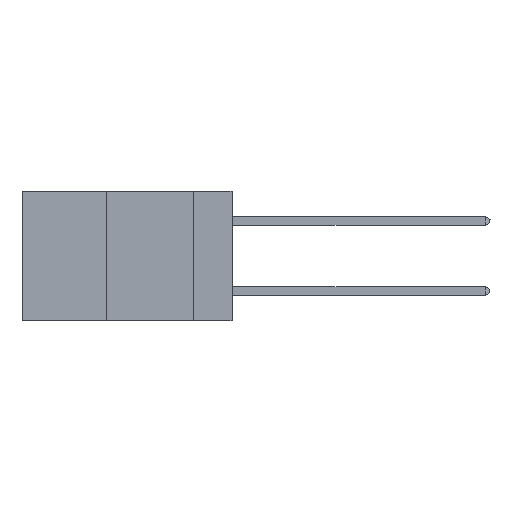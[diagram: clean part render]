
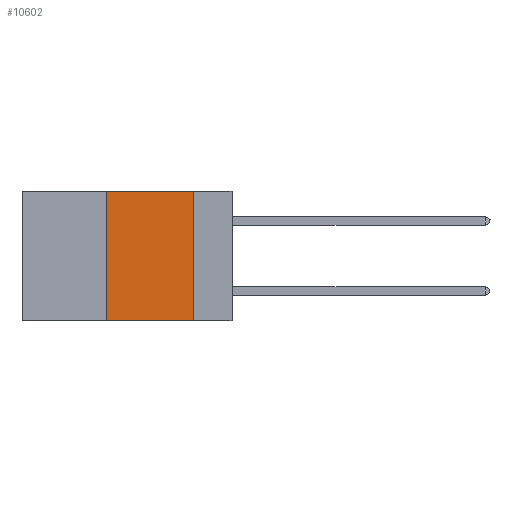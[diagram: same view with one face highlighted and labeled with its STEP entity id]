
A CAD part, left-side view. The second image highlights one B-rep face of the part: STEP entity #10602.
In plain terms, the highlighted planar face has unit normal (-1, 0, 0).
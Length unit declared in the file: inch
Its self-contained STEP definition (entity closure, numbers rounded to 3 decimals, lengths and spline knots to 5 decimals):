
#455 = VERTEX_POINT ( 'NONE', #4511 ) ;
#636 = EDGE_CURVE ( 'NONE', #7800, #2346, #3823, .T. ) ;
#637 = ORIENTED_EDGE ( 'NONE', *, *, #636, .F. ) ;
#1502 = EDGE_CURVE ( 'NONE', #5309, #455, #9808, .T. ) ;
#1651 = VECTOR ( 'NONE', #9748, 39.37008 ) ;
#1657 = DIRECTION ( 'NONE',  ( 0., 0., -1. ) ) ;
#1975 = ORIENTED_EDGE ( 'NONE', *, *, #7370, .F. ) ;
#2223 = ORIENTED_EDGE ( 'NONE', *, *, #1502, .F. ) ;
#2335 = CARTESIAN_POINT ( 'NONE',  ( 0., 0.36, -0.37 ) ) ;
#2346 = VERTEX_POINT ( 'NONE', #7310 ) ;
#2947 = DIRECTION ( 'NONE',  ( 0., 0., -1. ) ) ;
#3138 = CARTESIAN_POINT ( 'NONE',  ( 0., 0.11, 0. ) ) ;
#3528 = CARTESIAN_POINT ( 'NONE',  ( 0., 0.6, -0.37 ) ) ;
#3614 = FACE_OUTER_BOUND ( 'NONE', #5863, .T. ) ;
#3823 = LINE ( 'NONE', #5460, #9038 ) ;
#4129 = LINE ( 'NONE', #3528, #1651 ) ;
#4413 = CARTESIAN_POINT ( 'NONE',  ( 0., 0.36, 0. ) ) ;
#4511 = CARTESIAN_POINT ( 'NONE',  ( 0., 0.36, 0. ) ) ;
#5309 = VERTEX_POINT ( 'NONE', #2335 ) ;
#5460 = CARTESIAN_POINT ( 'NONE',  ( 0., 0.11, 0. ) ) ;
#5483 = ORIENTED_EDGE ( 'NONE', *, *, #10167, .T. ) ;
#5630 = CARTESIAN_POINT ( 'NONE',  ( 0., 0.6, 0. ) ) ;
#5693 = AXIS2_PLACEMENT_3D ( 'NONE', #6586, #10315, #1657 ) ;
#5863 = EDGE_LOOP ( 'NONE', ( #637, #1975, #2223, #5483 ) ) ;
#6318 = LINE ( 'NONE', #5630, #10533 ) ;
#6586 = CARTESIAN_POINT ( 'NONE',  ( 0., 0.6, 0. ) ) ;
#6979 = DIRECTION ( 'NONE',  ( 0., -1., 0. ) ) ;
#7310 = CARTESIAN_POINT ( 'NONE',  ( 0., 0.11, -0.37 ) ) ;
#7370 = EDGE_CURVE ( 'NONE', #455, #7800, #6318, .T. ) ;
#7800 = VERTEX_POINT ( 'NONE', #3138 ) ;
#7964 = DIRECTION ( 'NONE',  ( 0., 0., 1. ) ) ;
#9038 = VECTOR ( 'NONE', #2947, 39.37008 ) ;
#9137 = VECTOR ( 'NONE', #7964, 39.37008 ) ;
#9748 = DIRECTION ( 'NONE',  ( 0., -1., 0. ) ) ;
#9808 = LINE ( 'NONE', #4413, #9137 ) ;
#10167 = EDGE_CURVE ( 'NONE', #5309, #2346, #4129, .T. ) ;
#10315 = DIRECTION ( 'NONE',  ( 1., 0., 0. ) ) ;
#10533 = VECTOR ( 'NONE', #6979, 39.37008 ) ;
#10602 = ADVANCED_FACE ( 'NONE', ( #3614 ), #10980, .F. ) ;
#10980 = PLANE ( 'NONE',  #5693 ) ;
